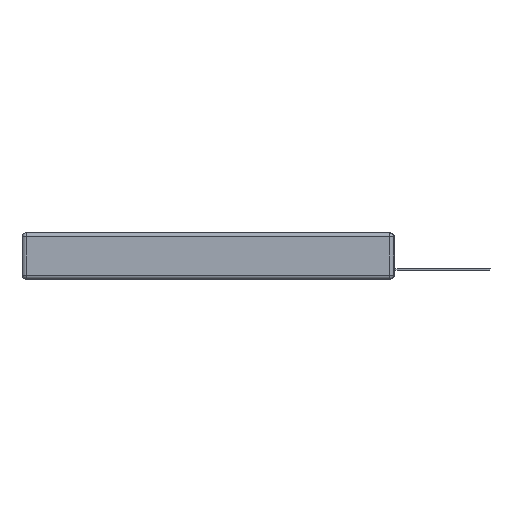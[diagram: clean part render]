
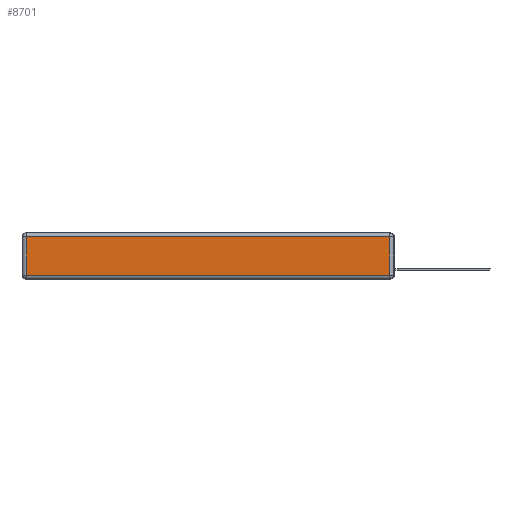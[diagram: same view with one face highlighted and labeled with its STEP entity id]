
A CAD part, left-side view. The second image highlights one B-rep face of the part: STEP entity #8701.
In plain terms, the highlighted planar face has unit normal (-1, 0, 0).
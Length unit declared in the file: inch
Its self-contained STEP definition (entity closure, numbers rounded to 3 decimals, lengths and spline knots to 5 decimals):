
#667 = VERTEX_POINT ( 'NONE', #8283 ) ;
#1279 = ORIENTED_EDGE ( 'NONE', *, *, #4534, .T. ) ;
#1855 = ORIENTED_EDGE ( 'NONE', *, *, #14003, .T. ) ;
#2071 = CARTESIAN_POINT ( 'NONE',  ( 0., 0., -0.343 ) ) ;
#2577 = LINE ( 'NONE', #19902, #12947 ) ;
#3286 = VECTOR ( 'NONE', #11399, 39.37008 ) ;
#3295 = CARTESIAN_POINT ( 'NONE',  ( 0., 0.03, -0.03 ) ) ;
#3486 = LINE ( 'NONE', #8420, #5389 ) ;
#3549 = PLANE ( 'NONE',  #7293 ) ;
#4448 = ORIENTED_EDGE ( 'NONE', *, *, #7285, .T. ) ;
#4534 = EDGE_CURVE ( 'NONE', #19608, #667, #2577, .T. ) ;
#5389 = VECTOR ( 'NONE', #17817, 39.37008 ) ;
#5561 = LINE ( 'NONE', #12069, #7356 ) ;
#5942 = VERTEX_POINT ( 'NONE', #3295 ) ;
#6545 = VERTEX_POINT ( 'NONE', #15040 ) ;
#6617 = LINE ( 'NONE', #10030, #3286 ) ;
#7285 = EDGE_CURVE ( 'NONE', #6545, #5942, #6617, .T. ) ;
#7293 = AXIS2_PLACEMENT_3D ( 'NONE', #2071, #8379, #11795 ) ;
#7356 = VECTOR ( 'NONE', #10506, 39.37008 ) ;
#8283 = CARTESIAN_POINT ( 'NONE',  ( 0., 2.72, -0.313 ) ) ;
#8379 = DIRECTION ( 'NONE',  ( -1., 0., 0. ) ) ;
#8420 = CARTESIAN_POINT ( 'NONE',  ( 0., 0., -0.313 ) ) ;
#8701 = ADVANCED_FACE ( 'NONE', ( #17692 ), #3549, .T. ) ;
#9783 = EDGE_LOOP ( 'NONE', ( #1855, #4448, #19712, #1279 ) ) ;
#10030 = CARTESIAN_POINT ( 'NONE',  ( 0., 0.03, -0.343 ) ) ;
#10506 = DIRECTION ( 'NONE',  ( 0., 1., 0. ) ) ;
#11399 = DIRECTION ( 'NONE',  ( 0., 0., 1. ) ) ;
#11795 = DIRECTION ( 'NONE',  ( 0., 0., 1. ) ) ;
#12069 = CARTESIAN_POINT ( 'NONE',  ( 0., 2.75, -0.03 ) ) ;
#12947 = VECTOR ( 'NONE', #15460, 39.37008 ) ;
#14003 = EDGE_CURVE ( 'NONE', #667, #6545, #3486, .T. ) ;
#15040 = CARTESIAN_POINT ( 'NONE',  ( 0., 0.03, -0.313 ) ) ;
#15460 = DIRECTION ( 'NONE',  ( 0., 0., -1. ) ) ;
#16498 = CARTESIAN_POINT ( 'NONE',  ( 0., 2.72, -0.03 ) ) ;
#16538 = EDGE_CURVE ( 'NONE', #5942, #19608, #5561, .T. ) ;
#17692 = FACE_OUTER_BOUND ( 'NONE', #9783, .T. ) ;
#17817 = DIRECTION ( 'NONE',  ( 0., -1., 0. ) ) ;
#19608 = VERTEX_POINT ( 'NONE', #16498 ) ;
#19712 = ORIENTED_EDGE ( 'NONE', *, *, #16538, .T. ) ;
#19902 = CARTESIAN_POINT ( 'NONE',  ( 0., 2.72, -0.343 ) ) ;
